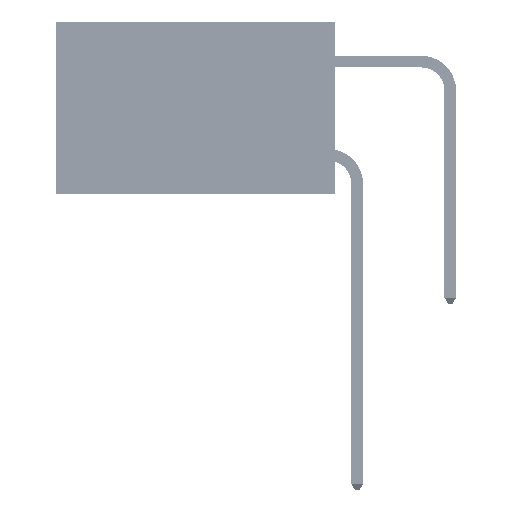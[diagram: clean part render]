
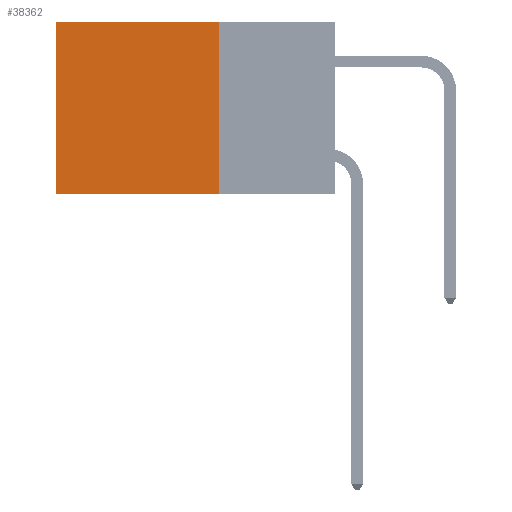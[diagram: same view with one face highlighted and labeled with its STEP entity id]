
A CAD part, left-side view. The second image highlights one B-rep face of the part: STEP entity #38362.
In plain terms, the highlighted planar face has unit normal (-1, 0, 0).
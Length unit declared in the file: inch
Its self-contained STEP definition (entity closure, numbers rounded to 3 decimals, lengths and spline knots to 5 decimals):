
#1386 = VECTOR ( 'NONE', #24136, 39.37008 ) ;
#2035 = ORIENTED_EDGE ( 'NONE', *, *, #4191, .F. ) ;
#3380 = DIRECTION ( 'NONE',  ( 1., 0., 0. ) ) ;
#4191 = EDGE_CURVE ( 'NONE', #31894, #18803, #17398, .T. ) ;
#5537 = CARTESIAN_POINT ( 'NONE',  ( 0.2875, 0.6, 0. ) ) ;
#9884 = CARTESIAN_POINT ( 'NONE',  ( 0.2875, 0.25, 0. ) ) ;
#12187 = EDGE_CURVE ( 'NONE', #31894, #30677, #41861, .T. ) ;
#13512 = EDGE_LOOP ( 'NONE', ( #34810, #42271, #2035, #29884 ) ) ;
#17338 = AXIS2_PLACEMENT_3D ( 'NONE', #35372, #3380, #27910 ) ;
#17398 = LINE ( 'NONE', #35146, #25989 ) ;
#18173 = VERTEX_POINT ( 'NONE', #29334 ) ;
#18803 = VERTEX_POINT ( 'NONE', #42985 ) ;
#19776 = DIRECTION ( 'NONE',  ( 0., 0., -1. ) ) ;
#20910 = DIRECTION ( 'NONE',  ( 0., 0., -1. ) ) ;
#23365 = CARTESIAN_POINT ( 'NONE',  ( 0.2875, 0.25, -0.37 ) ) ;
#23830 = DIRECTION ( 'NONE',  ( 0., 1., 0. ) ) ;
#24136 = DIRECTION ( 'NONE',  ( 0., 1., 0. ) ) ;
#25238 = CARTESIAN_POINT ( 'NONE',  ( 0.2875, 0.25, 0. ) ) ;
#25649 = VECTOR ( 'NONE', #23830, 39.37008 ) ;
#25660 = EDGE_CURVE ( 'NONE', #18803, #18173, #37362, .T. ) ;
#25776 = VECTOR ( 'NONE', #19776, 39.37008 ) ;
#25989 = VECTOR ( 'NONE', #20910, 39.37008 ) ;
#27380 = EDGE_CURVE ( 'NONE', #30677, #18173, #41026, .T. ) ;
#27910 = DIRECTION ( 'NONE',  ( 0., 0., -1. ) ) ;
#29334 = CARTESIAN_POINT ( 'NONE',  ( 0.2875, 0.6, -0.37 ) ) ;
#29884 = ORIENTED_EDGE ( 'NONE', *, *, #12187, .T. ) ;
#30677 = VERTEX_POINT ( 'NONE', #45291 ) ;
#31633 = FACE_OUTER_BOUND ( 'NONE', #13512, .T. ) ;
#31894 = VERTEX_POINT ( 'NONE', #25238 ) ;
#34810 = ORIENTED_EDGE ( 'NONE', *, *, #27380, .T. ) ;
#35146 = CARTESIAN_POINT ( 'NONE',  ( 0.2875, 0.25, 0. ) ) ;
#35372 = CARTESIAN_POINT ( 'NONE',  ( 0.2875, 0.25, 0. ) ) ;
#37362 = LINE ( 'NONE', #23365, #25649 ) ;
#38362 = ADVANCED_FACE ( 'NONE', ( #31633 ), #45410, .F. ) ;
#41026 = LINE ( 'NONE', #5537, #25776 ) ;
#41861 = LINE ( 'NONE', #9884, #1386 ) ;
#42271 = ORIENTED_EDGE ( 'NONE', *, *, #25660, .F. ) ;
#42985 = CARTESIAN_POINT ( 'NONE',  ( 0.2875, 0.25, -0.37 ) ) ;
#45291 = CARTESIAN_POINT ( 'NONE',  ( 0.2875, 0.6, 0. ) ) ;
#45410 = PLANE ( 'NONE',  #17338 ) ;
